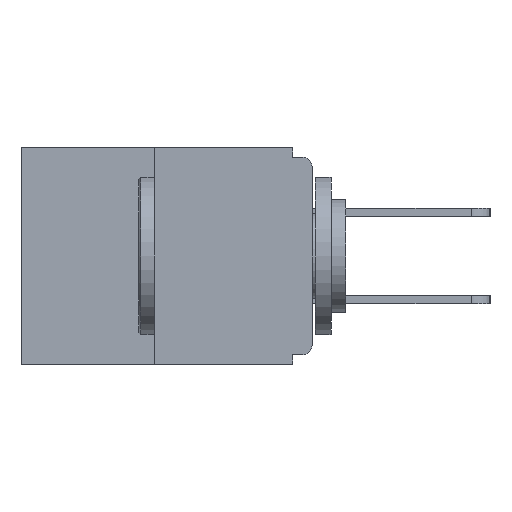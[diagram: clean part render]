
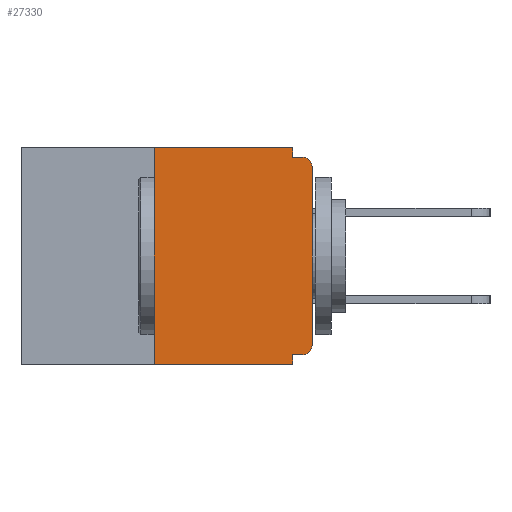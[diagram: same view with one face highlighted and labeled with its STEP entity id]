
A CAD part, left-side view. The second image highlights one B-rep face of the part: STEP entity #27330.
In plain terms, the highlighted planar face has unit normal (-1, 0, 0).
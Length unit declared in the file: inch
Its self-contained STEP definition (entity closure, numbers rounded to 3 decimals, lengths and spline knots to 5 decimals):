
#511 = CARTESIAN_POINT ( 'NONE',  ( 0., 0.46, 0. ) ) ;
#555 = DIRECTION ( 'NONE',  ( 0., -1., 0. ) ) ;
#847 = CARTESIAN_POINT ( 'NONE',  ( 0., 0.46, -0.343 ) ) ;
#1564 = VERTEX_POINT ( 'NONE', #15360 ) ;
#1800 = CARTESIAN_POINT ( 'NONE',  ( 0., 0.031, -0.343 ) ) ;
#2052 = AXIS2_PLACEMENT_3D ( 'NONE', #511, #5217, #21567 ) ;
#2254 = EDGE_CURVE ( 'NONE', #12235, #8633, #19673, .T. ) ;
#2362 = CARTESIAN_POINT ( 'NONE',  ( 0., 0.031, 0. ) ) ;
#2848 = CARTESIAN_POINT ( 'NONE',  ( 0., 0.031, -0.328 ) ) ;
#3620 = EDGE_CURVE ( 'NONE', #1564, #21772, #4301, .T. ) ;
#3973 = EDGE_CURVE ( 'NONE', #20376, #28513, #14168, .T. ) ;
#4138 = DIRECTION ( 'NONE',  ( 0., 0., -1. ) ) ;
#4301 = LINE ( 'NONE', #7514, #17431 ) ;
#4489 = DIRECTION ( 'NONE',  ( 0., 0., -1. ) ) ;
#4694 = CARTESIAN_POINT ( 'NONE',  ( 0., 0., -0.313 ) ) ;
#5217 = DIRECTION ( 'NONE',  ( 1., 0., 0. ) ) ;
#5647 = ORIENTED_EDGE ( 'NONE', *, *, #3620, .F. ) ;
#7514 = CARTESIAN_POINT ( 'NONE',  ( 0., 0.25, 0. ) ) ;
#7616 = DIRECTION ( 'NONE',  ( 0., 0., 1. ) ) ;
#7656 = CARTESIAN_POINT ( 'NONE',  ( 0., 0., -0.328 ) ) ;
#7761 = CARTESIAN_POINT ( 'NONE',  ( 0., 0., -0.015 ) ) ;
#7865 = EDGE_LOOP ( 'NONE', ( #18610, #5647, #24447, #15149, #13535, #22365, #12757, #22097, #15502, #8571 ) ) ;
#8571 = ORIENTED_EDGE ( 'NONE', *, *, #3973, .F. ) ;
#8599 = EDGE_CURVE ( 'NONE', #8633, #14030, #13903, .T. ) ;
#8633 = VERTEX_POINT ( 'NONE', #4694 ) ;
#8776 = VERTEX_POINT ( 'NONE', #2848 ) ;
#10419 = FACE_OUTER_BOUND ( 'NONE', #7865, .T. ) ;
#10691 = VECTOR ( 'NONE', #555, 39.37008 ) ;
#11669 = CARTESIAN_POINT ( 'NONE',  ( 0., 0.015, -0.313 ) ) ;
#12235 = VERTEX_POINT ( 'NONE', #24972 ) ;
#12431 = VECTOR ( 'NONE', #23099, 39.37008 ) ;
#12491 = VECTOR ( 'NONE', #24104, 39.37008 ) ;
#12662 = EDGE_CURVE ( 'NONE', #1564, #15907, #27805, .T. ) ;
#12757 = ORIENTED_EDGE ( 'NONE', *, *, #8599, .T. ) ;
#12771 = CARTESIAN_POINT ( 'NONE',  ( 0., 0.031, 0. ) ) ;
#13535 = ORIENTED_EDGE ( 'NONE', *, *, #25316, .F. ) ;
#13839 = VECTOR ( 'NONE', #14408, 39.37008 ) ;
#13903 = LINE ( 'NONE', #27370, #12431 ) ;
#13913 = DIRECTION ( 'NONE',  ( -1., 0., 0. ) ) ;
#14030 = VERTEX_POINT ( 'NONE', #28598 ) ;
#14168 = LINE ( 'NONE', #2362, #27635 ) ;
#14408 = DIRECTION ( 'NONE',  ( 0., 1., 0. ) ) ;
#14977 = VECTOR ( 'NONE', #4138, 39.37008 ) ;
#15023 = EDGE_CURVE ( 'NONE', #14030, #16985, #24002, .T. ) ;
#15149 = ORIENTED_EDGE ( 'NONE', *, *, #23704, .F. ) ;
#15360 = CARTESIAN_POINT ( 'NONE',  ( 0., 0.25, -0.343 ) ) ;
#15502 = ORIENTED_EDGE ( 'NONE', *, *, #22855, .F. ) ;
#15907 = VERTEX_POINT ( 'NONE', #29617 ) ;
#16040 = LINE ( 'NONE', #1800, #14977 ) ;
#16457 = DIRECTION ( 'NONE',  ( 0., 0., -1. ) ) ;
#16985 = VERTEX_POINT ( 'NONE', #19653 ) ;
#17431 = VECTOR ( 'NONE', #7616, 39.37008 ) ;
#18610 = ORIENTED_EDGE ( 'NONE', *, *, #18731, .F. ) ;
#18731 = EDGE_CURVE ( 'NONE', #21772, #20376, #21514, .T. ) ;
#18748 = DIRECTION ( 'NONE',  ( 0., 0., -1. ) ) ;
#19653 = CARTESIAN_POINT ( 'NONE',  ( 0., 0.015, -0.015 ) ) ;
#19673 = CIRCLE ( 'NONE', #22781, 0.015 ) ;
#20376 = VERTEX_POINT ( 'NONE', #12771 ) ;
#21155 = AXIS2_PLACEMENT_3D ( 'NONE', #27955, #25523, #18748 ) ;
#21514 = LINE ( 'NONE', #23673, #28078 ) ;
#21567 = DIRECTION ( 'NONE',  ( 0., 0., -1. ) ) ;
#21772 = VERTEX_POINT ( 'NONE', #26729 ) ;
#22097 = ORIENTED_EDGE ( 'NONE', *, *, #15023, .T. ) ;
#22365 = ORIENTED_EDGE ( 'NONE', *, *, #2254, .T. ) ;
#22781 = AXIS2_PLACEMENT_3D ( 'NONE', #11669, #13913, #4489 ) ;
#22855 = EDGE_CURVE ( 'NONE', #28513, #16985, #28162, .T. ) ;
#23099 = DIRECTION ( 'NONE',  ( 0., 0., 1. ) ) ;
#23673 = CARTESIAN_POINT ( 'NONE',  ( 0., 0.46, 0. ) ) ;
#23704 = EDGE_CURVE ( 'NONE', #8776, #15907, #16040, .T. ) ;
#24002 = CIRCLE ( 'NONE', #21155, 0.015 ) ;
#24104 = DIRECTION ( 'NONE',  ( 0., -1., 0. ) ) ;
#24447 = ORIENTED_EDGE ( 'NONE', *, *, #12662, .T. ) ;
#24972 = CARTESIAN_POINT ( 'NONE',  ( 0., 0.015, -0.328 ) ) ;
#25316 = EDGE_CURVE ( 'NONE', #12235, #8776, #27692, .T. ) ;
#25523 = DIRECTION ( 'NONE',  ( -1., 0., 0. ) ) ;
#26690 = DIRECTION ( 'NONE',  ( 0., -1., 0. ) ) ;
#26729 = CARTESIAN_POINT ( 'NONE',  ( 0., 0.25, 0. ) ) ;
#27330 = ADVANCED_FACE ( 'NONE', ( #10419 ), #28489, .F. ) ;
#27370 = CARTESIAN_POINT ( 'NONE',  ( 0., 0., 0. ) ) ;
#27635 = VECTOR ( 'NONE', #16457, 39.37008 ) ;
#27692 = LINE ( 'NONE', #7656, #13839 ) ;
#27805 = LINE ( 'NONE', #847, #10691 ) ;
#27955 = CARTESIAN_POINT ( 'NONE',  ( 0., 0.015, -0.03 ) ) ;
#27960 = CARTESIAN_POINT ( 'NONE',  ( 0., 0.031, -0.015 ) ) ;
#28078 = VECTOR ( 'NONE', #26690, 39.37008 ) ;
#28162 = LINE ( 'NONE', #7761, #12491 ) ;
#28489 = PLANE ( 'NONE',  #2052 ) ;
#28513 = VERTEX_POINT ( 'NONE', #27960 ) ;
#28598 = CARTESIAN_POINT ( 'NONE',  ( 0., 0., -0.03 ) ) ;
#29617 = CARTESIAN_POINT ( 'NONE',  ( 0., 0.031, -0.343 ) ) ;
